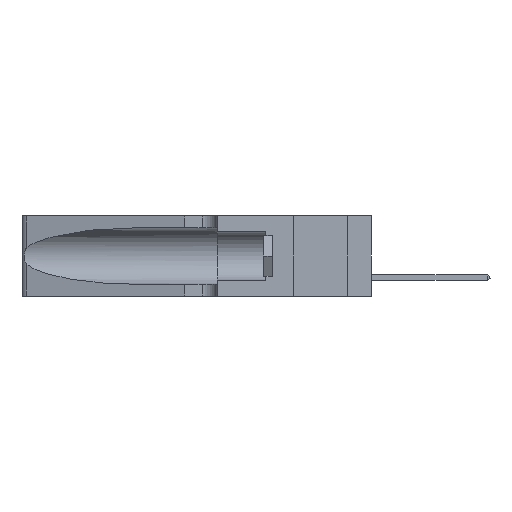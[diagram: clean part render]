
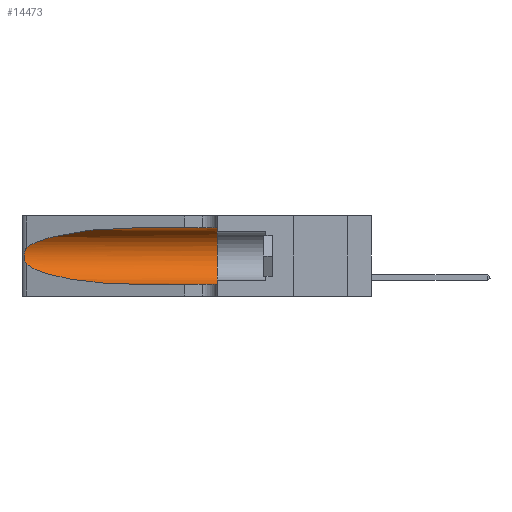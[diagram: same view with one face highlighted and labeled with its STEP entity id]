
A CAD part, left-side view. The second image highlights one B-rep face of the part: STEP entity #14473.
In plain terms, the highlighted cylindrical face has radius 3.308 mm (diameter 6.617 mm), a partial arc.
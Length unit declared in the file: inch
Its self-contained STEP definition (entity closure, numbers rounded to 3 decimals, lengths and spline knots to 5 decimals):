
#685 = EDGE_CURVE ( 'NONE', #8833, #23441, #12940, .T. ) ;
#974 = CARTESIAN_POINT ( 'NONE',  ( 0.25639, 1.23184, 0.21858 ) ) ;
#1064 = CARTESIAN_POINT ( 'NONE',  ( 0.25487, 1.22718, 0.22369 ) ) ;
#1641 = CARTESIAN_POINT ( 'NONE',  ( 0.25487, 1.22718, 0.14631 ) ) ;
#2240 = VERTEX_POINT ( 'NONE', #15080 ) ;
#2317 = VERTEX_POINT ( 'NONE', #8096 ) ;
#2577 = CARTESIAN_POINT ( 'NONE',  ( 0.1305, 1.61858, 0.31525 ) ) ;
#2636 = CARTESIAN_POINT ( 'NONE',  ( 0.25487, 1.22718, 0.14631 ) ) ;
#3445 = DIRECTION ( 'NONE',  ( 0., 0., -1. ) ) ;
#3959 =( BOUNDED_CURVE ( )  B_SPLINE_CURVE ( 3, ( #13202, #26914, #11518, #22784 ),
 .UNSPECIFIED., .F., .F. ) 
 B_SPLINE_CURVE_WITH_KNOTS ( ( 4, 4 ),
 ( 1.5708, 2.84003 ),
 .UNSPECIFIED. ) 
 CURVE ( )  GEOMETRIC_REPRESENTATION_ITEM ( )  RATIONAL_B_SPLINE_CURVE ( ( 1., 0.87, 0.87, 1. ) ) 
 REPRESENTATION_ITEM ( '' )  );
#4559 = VECTOR ( 'NONE', #9140, 39.37008 ) ;
#4946 = FACE_OUTER_BOUND ( 'NONE', #23977, .T. ) ;
#5232 = EDGE_CURVE ( 'NONE', #11397, #20737, #10523, .T. ) ;
#5611 = CIRCLE ( 'NONE', #22484, 0.13025 ) ;
#5907 = CARTESIAN_POINT ( 'NONE',  ( 0.25789, 1.23486, 0.15765 ) ) ;
#5971 = CARTESIAN_POINT ( 'NONE',  ( 0.1305, 1.61858, 0.05475 ) ) ;
#7314 = VECTOR ( 'NONE', #14597, 39.37008 ) ;
#7683 = CARTESIAN_POINT ( 'NONE',  ( 0.26018, 1.23835, 0.19895 ) ) ;
#7952 = CARTESIAN_POINT ( 'NONE',  ( 0.1305, 0.72297, 0.05475 ) ) ;
#8096 = CARTESIAN_POINT ( 'NONE',  ( 0.25487, 1.22718, 0.22369 ) ) ;
#8833 = VERTEX_POINT ( 'NONE', #28975 ) ;
#9140 = DIRECTION ( 'NONE',  ( 0., -1., 0. ) ) ;
#9524 = ORIENTED_EDGE ( 'NONE', *, *, #28059, .T. ) ;
#9600 = ORIENTED_EDGE ( 'NONE', *, *, #18136, .T. ) ;
#10041 = CARTESIAN_POINT ( 'NONE',  ( 0.25856, 1.23593, 0.16098 ) ) ;
#10523 = LINE ( 'NONE', #2577, #4559 ) ;
#10677 = CARTESIAN_POINT ( 'NONE',  ( 0.1305, 0.35, 0.185 ) ) ;
#11397 = VERTEX_POINT ( 'NONE', #12754 ) ;
#11518 = CARTESIAN_POINT ( 'NONE',  ( 0.2373, 1.15595, 0.28018 ) ) ;
#11640 = ORIENTED_EDGE ( 'NONE', *, *, #5232, .F. ) ;
#12754 = CARTESIAN_POINT ( 'NONE',  ( 0.1305, 0.72297, 0.31525 ) ) ;
#12940 =( BOUNDED_CURVE ( )  B_SPLINE_CURVE ( 3, ( #2636, #18521, #13872, #25251 ),
 .UNSPECIFIED., .F., .F. ) 
 B_SPLINE_CURVE_WITH_KNOTS ( ( 4, 4 ),
 ( 3.44316, 4.71239 ),
 .UNSPECIFIED. ) 
 CURVE ( )  GEOMETRIC_REPRESENTATION_ITEM ( )  RATIONAL_B_SPLINE_CURVE ( ( 1., 0.87, 0.87, 1. ) ) 
 REPRESENTATION_ITEM ( '' )  );
#13202 = CARTESIAN_POINT ( 'NONE',  ( 0.1305, 0.72297, 0.31525 ) ) ;
#13872 = CARTESIAN_POINT ( 'NONE',  ( 0.18966, 0.96281, 0.05475 ) ) ;
#14420 = AXIS2_PLACEMENT_3D ( 'NONE', #26171, #19438, #3445 ) ;
#14435 = ORIENTED_EDGE ( 'NONE', *, *, #685, .T. ) ;
#14473 = ADVANCED_FACE ( 'NONE', ( #4946 ), #25272, .F. ) ;
#14529 = EDGE_CURVE ( 'NONE', #23441, #2240, #19971, .T. ) ;
#14597 = DIRECTION ( 'NONE',  ( 0., -1., 0. ) ) ;
#15080 = CARTESIAN_POINT ( 'NONE',  ( 0.1305, 0.35, 0.05475 ) ) ;
#18136 = EDGE_CURVE ( 'NONE', #2317, #8833, #19607, .T. ) ;
#18445 = ORIENTED_EDGE ( 'NONE', *, *, #14529, .T. ) ;
#18521 = CARTESIAN_POINT ( 'NONE',  ( 0.2373, 1.15595, 0.08982 ) ) ;
#18890 = CARTESIAN_POINT ( 'NONE',  ( 0.25787, 1.23484, 0.2124 ) ) ;
#18989 = CARTESIAN_POINT ( 'NONE',  ( 0.25555, 1.22994, 0.2215 ) ) ;
#19178 = CARTESIAN_POINT ( 'NONE',  ( 0.25555, 1.22993, 0.14849 ) ) ;
#19438 = DIRECTION ( 'NONE',  ( 0., -1., 0. ) ) ;
#19607 = B_SPLINE_CURVE_WITH_KNOTS ( 'NONE', 3,
 ( #1064, #18989, #974, #18890, #21127, #7683, #28057, #21227, #23347, #10041, #5907, #23739, #19178, #1641 ),
 .UNSPECIFIED., .F., .F.,
 ( 4, 2, 2, 2, 2, 2, 4 ),
 ( 0., 0.00027, 0.00053, 0.00107, 0.0016, 0.00187, 0.00214 ),
 .UNSPECIFIED. ) ;
#19971 = LINE ( 'NONE', #5971, #7314 ) ;
#20737 = VERTEX_POINT ( 'NONE', #21175 ) ;
#21127 = CARTESIAN_POINT ( 'NONE',  ( 0.25854, 1.2359, 0.20912 ) ) ;
#21163 = ORIENTED_EDGE ( 'NONE', *, *, #22782, .F. ) ;
#21175 = CARTESIAN_POINT ( 'NONE',  ( 0.1305, 0.35, 0.31525 ) ) ;
#21227 = CARTESIAN_POINT ( 'NONE',  ( 0.26075, 1.23896, 0.178 ) ) ;
#22484 = AXIS2_PLACEMENT_3D ( 'NONE', #10677, #26361, #24273 ) ;
#22782 = EDGE_CURVE ( 'NONE', #20737, #2240, #5611, .T. ) ;
#22784 = CARTESIAN_POINT ( 'NONE',  ( 0.25487, 1.22718, 0.22369 ) ) ;
#23347 = CARTESIAN_POINT ( 'NONE',  ( 0.26017, 1.23833, 0.17102 ) ) ;
#23441 = VERTEX_POINT ( 'NONE', #7952 ) ;
#23739 = CARTESIAN_POINT ( 'NONE',  ( 0.25639, 1.23186, 0.15144 ) ) ;
#23977 = EDGE_LOOP ( 'NONE', ( #9524, #9600, #14435, #18445, #21163, #11640 ) ) ;
#24273 = DIRECTION ( 'NONE',  ( 0., 0., 1. ) ) ;
#25251 = CARTESIAN_POINT ( 'NONE',  ( 0.1305, 0.72297, 0.05475 ) ) ;
#25272 = CYLINDRICAL_SURFACE ( 'NONE', #14420, 0.13025 ) ;
#26171 = CARTESIAN_POINT ( 'NONE',  ( 0.1305, 1.61858, 0.185 ) ) ;
#26361 = DIRECTION ( 'NONE',  ( 0., 1., 0. ) ) ;
#26914 = CARTESIAN_POINT ( 'NONE',  ( 0.18966, 0.96281, 0.31525 ) ) ;
#28057 = CARTESIAN_POINT ( 'NONE',  ( 0.26075, 1.23896, 0.19203 ) ) ;
#28059 = EDGE_CURVE ( 'NONE', #11397, #2317, #3959, .T. ) ;
#28975 = CARTESIAN_POINT ( 'NONE',  ( 0.25487, 1.22718, 0.14631 ) ) ;
